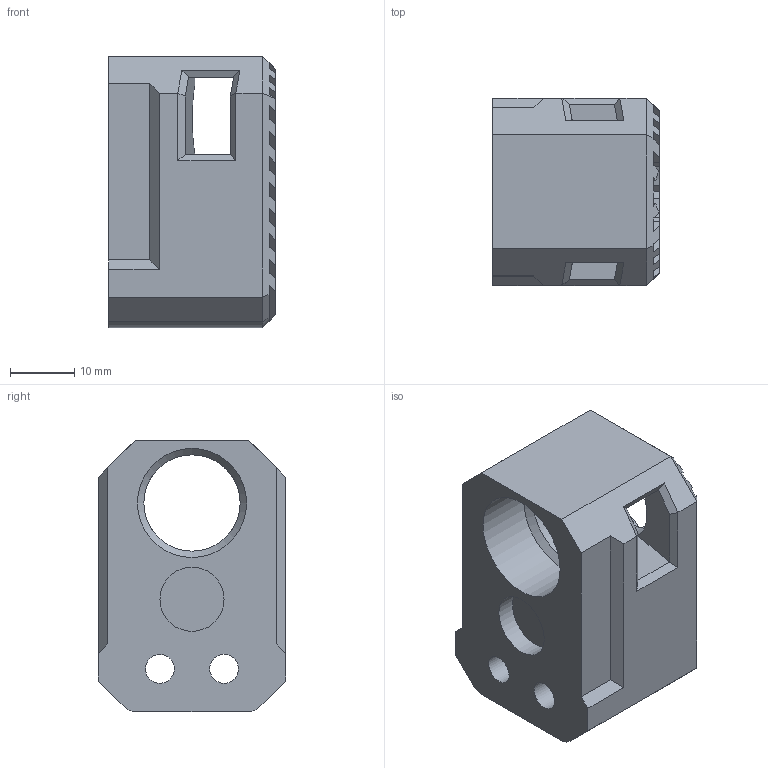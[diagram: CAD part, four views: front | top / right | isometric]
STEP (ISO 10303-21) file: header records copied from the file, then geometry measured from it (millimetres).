
FILE_DESCRIPTION(/* description */ (''),/* implementation_level */ '2;1');
FILE_NAME(/* name */ 'CRUSHER COMP.step',/* time_stamp */ '2022-07-31T11:38:35-05:00',/* author */ (''),/* organization */ (''),/* preprocessor_version */ 'ST-DEVELOPER v19',/* originating_system */ 'Autodesk Translation Framework v11.7.0.108',/* authorisation */ '');
FILE_SCHEMA (('AUTOMOTIVE_DESIGN { 1 0 10303 214 3 1 1 }'));
Length unit declared in the file: millimetre
Products named in the file (1): PY2A SDI GXL CRUSHER
Bounding box: 26 x 29.23 x 42.25 mm (x, y, z)
Volume: 21620 mm3; surface area: 7874.6 mm2
Topology: 1 solids, 1 shells, 187 faces, 519 edges, 332 vertices
Faces by surface type: plane 161, cylinder 22, cone 4
Full cylindrical faces by diameter (mm): 4.5 x2, 7.5 x2, 10 x1, 15 x1, 17 x1
Entity records: 5936 total; most frequent: CARTESIAN_POINT 1039, ORIENTED_EDGE 1038, DIRECTION 981, EDGE_CURVE 519, LINE 433, VECTOR 433, VERTEX_POINT 332, AXIS2_PLACEMENT_3D 274
